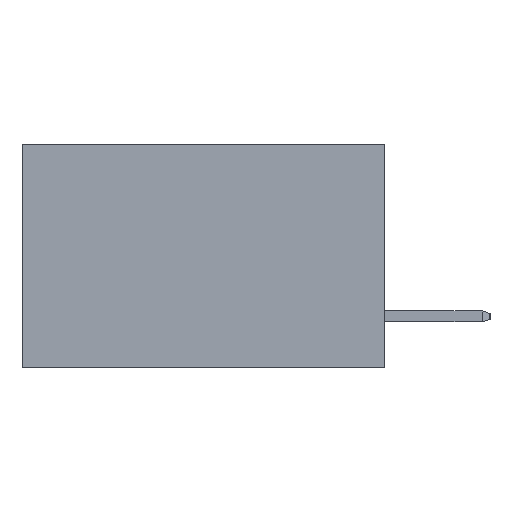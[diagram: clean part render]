
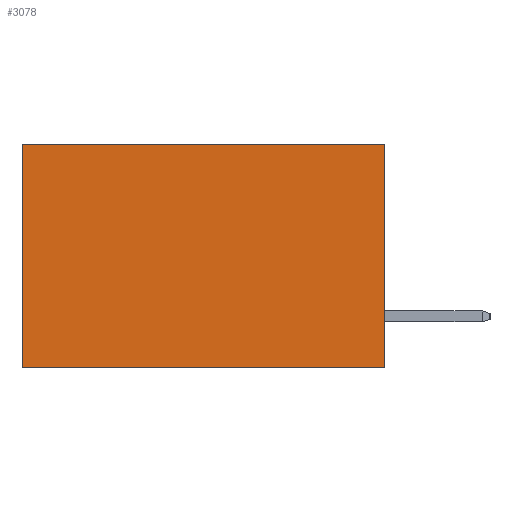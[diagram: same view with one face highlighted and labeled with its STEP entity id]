
A CAD part, left-side view. The second image highlights one B-rep face of the part: STEP entity #3078.
In plain terms, the highlighted planar face has unit normal (-1, 0, 0).
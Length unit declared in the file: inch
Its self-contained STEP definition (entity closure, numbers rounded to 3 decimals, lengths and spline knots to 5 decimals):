
#613 = VERTEX_POINT ( 'NONE', #4481 ) ;
#1160 = ORIENTED_EDGE ( 'NONE', *, *, #9667, .T. ) ;
#3078 = ADVANCED_FACE ( 'NONE', ( #13854 ), #14806, .F. ) ;
#4011 = CARTESIAN_POINT ( 'NONE',  ( 0.2615, 0., 0. ) ) ;
#4136 = LINE ( 'NONE', #5026, #7305 ) ;
#4481 = CARTESIAN_POINT ( 'NONE',  ( 0.2615, 0., 0. ) ) ;
#4621 = LINE ( 'NONE', #13864, #13591 ) ;
#5026 = CARTESIAN_POINT ( 'NONE',  ( 0.2615, 0., -0.37 ) ) ;
#5259 = CARTESIAN_POINT ( 'NONE',  ( 0.2615, 0.6, 0. ) ) ;
#5354 = AXIS2_PLACEMENT_3D ( 'NONE', #13916, #14158, #15162 ) ;
#5395 = EDGE_CURVE ( 'NONE', #613, #5889, #4621, .T. ) ;
#5416 = VECTOR ( 'NONE', #6428, 39.37008 ) ;
#5889 = VERTEX_POINT ( 'NONE', #10718 ) ;
#6428 = DIRECTION ( 'NONE',  ( 0., 1., 0. ) ) ;
#7305 = VECTOR ( 'NONE', #13211, 39.37008 ) ;
#7819 = VERTEX_POINT ( 'NONE', #5259 ) ;
#8635 = CARTESIAN_POINT ( 'NONE',  ( 0.2615, 0.6, -0.37 ) ) ;
#8901 = LINE ( 'NONE', #4011, #5416 ) ;
#9667 = EDGE_CURVE ( 'NONE', #7819, #13002, #13708, .T. ) ;
#9829 = DIRECTION ( 'NONE',  ( 0., 0., -1. ) ) ;
#10705 = EDGE_CURVE ( 'NONE', #5889, #13002, #4136, .T. ) ;
#10718 = CARTESIAN_POINT ( 'NONE',  ( 0.2615, 0., -0.37 ) ) ;
#11506 = ORIENTED_EDGE ( 'NONE', *, *, #12797, .T. ) ;
#12701 = CARTESIAN_POINT ( 'NONE',  ( 0.2615, 0.6, -0.37 ) ) ;
#12797 = EDGE_CURVE ( 'NONE', #613, #7819, #8901, .T. ) ;
#13002 = VERTEX_POINT ( 'NONE', #12701 ) ;
#13113 = EDGE_LOOP ( 'NONE', ( #1160, #13426, #13301, #11506 ) ) ;
#13211 = DIRECTION ( 'NONE',  ( 0., 1., 0. ) ) ;
#13301 = ORIENTED_EDGE ( 'NONE', *, *, #5395, .F. ) ;
#13349 = VECTOR ( 'NONE', #9829, 39.37008 ) ;
#13426 = ORIENTED_EDGE ( 'NONE', *, *, #10705, .F. ) ;
#13591 = VECTOR ( 'NONE', #13832, 39.37008 ) ;
#13708 = LINE ( 'NONE', #8635, #13349 ) ;
#13832 = DIRECTION ( 'NONE',  ( 0., 0., -1. ) ) ;
#13854 = FACE_OUTER_BOUND ( 'NONE', #13113, .T. ) ;
#13864 = CARTESIAN_POINT ( 'NONE',  ( 0.2615, 0., -0.37 ) ) ;
#13916 = CARTESIAN_POINT ( 'NONE',  ( 0.2615, 0., -0.37 ) ) ;
#14158 = DIRECTION ( 'NONE',  ( 1., 0., 0. ) ) ;
#14806 = PLANE ( 'NONE',  #5354 ) ;
#15162 = DIRECTION ( 'NONE',  ( 0., 0., -1. ) ) ;
